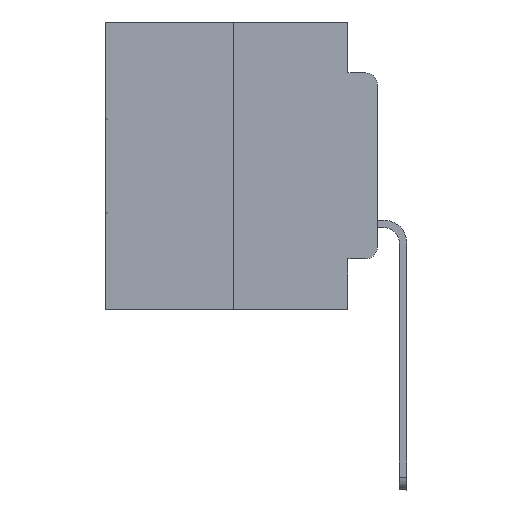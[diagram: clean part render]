
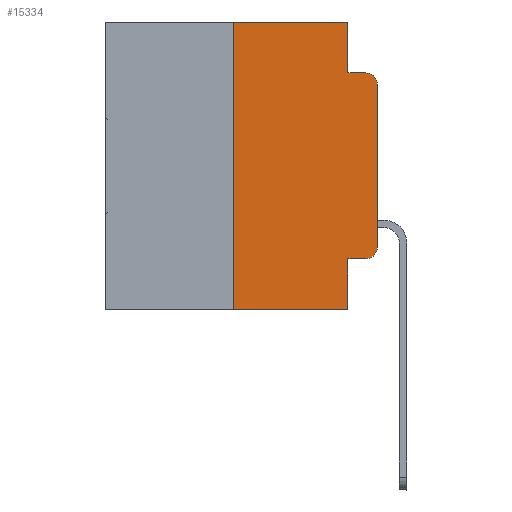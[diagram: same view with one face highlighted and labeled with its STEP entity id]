
A CAD part, left-side view. The second image highlights one B-rep face of the part: STEP entity #15334.
In plain terms, the highlighted planar face has unit normal (-1, 0, 0).
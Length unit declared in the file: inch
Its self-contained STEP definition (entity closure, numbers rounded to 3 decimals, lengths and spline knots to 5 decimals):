
#325 = AXIS2_PLACEMENT_3D ( 'NONE', #27544, #16345, #9337 ) ;
#445 = DIRECTION ( 'NONE',  ( 0., 0., -1. ) ) ;
#854 = CARTESIAN_POINT ( 'NONE',  ( 0., 0.051, -0.0885 ) ) ;
#1113 = DIRECTION ( 'NONE',  ( 1., 0., 0. ) ) ;
#1125 = VECTOR ( 'NONE', #6802, 39.37008 ) ;
#1430 = DIRECTION ( 'NONE',  ( 0., 0., -1. ) ) ;
#1581 = LINE ( 'NONE', #15450, #1125 ) ;
#1852 = VECTOR ( 'NONE', #19676, 39.37008 ) ;
#1858 = VECTOR ( 'NONE', #2871, 39.37008 ) ;
#1973 = CARTESIAN_POINT ( 'NONE',  ( 0., 0.051, -0.4115 ) ) ;
#2155 = EDGE_CURVE ( 'NONE', #29068, #17212, #22130, .T. ) ;
#2298 = EDGE_CURVE ( 'NONE', #24564, #20681, #26079, .T. ) ;
#2871 = DIRECTION ( 'NONE',  ( 0., -1., 0. ) ) ;
#3515 = PLANE ( 'NONE',  #11092 ) ;
#4290 = LINE ( 'NONE', #15476, #1852 ) ;
#4856 = DIRECTION ( 'NONE',  ( 0., -1., 0. ) ) ;
#5271 = CARTESIAN_POINT ( 'NONE',  ( 0., 0.02, -0.0885 ) ) ;
#5399 = CARTESIAN_POINT ( 'NONE',  ( 0., 0.051, -0.4115 ) ) ;
#5441 = CARTESIAN_POINT ( 'NONE',  ( 0., 0.25, -0.5 ) ) ;
#5605 = VECTOR ( 'NONE', #4856, 39.37008 ) ;
#6640 = EDGE_CURVE ( 'NONE', #12222, #18406, #27238, .T. ) ;
#6689 = EDGE_CURVE ( 'NONE', #25036, #13129, #12279, .T. ) ;
#6758 = VERTEX_POINT ( 'NONE', #5441 ) ;
#6802 = DIRECTION ( 'NONE',  ( 0., 0., -1. ) ) ;
#7118 = ORIENTED_EDGE ( 'NONE', *, *, #20360, .T. ) ;
#7338 = LINE ( 'NONE', #5399, #1858 ) ;
#7473 = ORIENTED_EDGE ( 'NONE', *, *, #18368, .F. ) ;
#7517 = CARTESIAN_POINT ( 'NONE',  ( 0., 0.473, -0.5 ) ) ;
#7795 = LINE ( 'NONE', #7517, #13905 ) ;
#8015 = CARTESIAN_POINT ( 'NONE',  ( 0., 0.051, 0. ) ) ;
#8665 = DIRECTION ( 'NONE',  ( 0., 0., -1. ) ) ;
#8822 = ORIENTED_EDGE ( 'NONE', *, *, #6640, .F. ) ;
#9126 = DIRECTION ( 'NONE',  ( 0., -1., 0. ) ) ;
#9337 = DIRECTION ( 'NONE',  ( 0., 0., -1. ) ) ;
#9690 = EDGE_CURVE ( 'NONE', #6758, #12222, #4290, .T. ) ;
#9694 = CARTESIAN_POINT ( 'NONE',  ( 0., 0.25, 0. ) ) ;
#9730 = CARTESIAN_POINT ( 'NONE',  ( 0., 0., -0.3915 ) ) ;
#11092 = AXIS2_PLACEMENT_3D ( 'NONE', #22046, #1113, #1430 ) ;
#11258 = AXIS2_PLACEMENT_3D ( 'NONE', #22275, #29105, #8665 ) ;
#11590 = CARTESIAN_POINT ( 'NONE',  ( 0., 0., -0.1085 ) ) ;
#11609 = VECTOR ( 'NONE', #9126, 39.37008 ) ;
#12222 = VERTEX_POINT ( 'NONE', #9694 ) ;
#12279 = CIRCLE ( 'NONE', #325, 0.02 ) ;
#12845 = ORIENTED_EDGE ( 'NONE', *, *, #20061, .T. ) ;
#13129 = VERTEX_POINT ( 'NONE', #9730 ) ;
#13905 = VECTOR ( 'NONE', #14505, 39.37008 ) ;
#13957 = CARTESIAN_POINT ( 'NONE',  ( 0., 0.051, -0.5 ) ) ;
#14182 = CARTESIAN_POINT ( 'NONE',  ( 0., 0., 0. ) ) ;
#14505 = DIRECTION ( 'NONE',  ( 0., -1., 0. ) ) ;
#14585 = VECTOR ( 'NONE', #28053, 39.37008 ) ;
#15334 = ADVANCED_FACE ( 'NONE', ( #19793 ), #3515, .F. ) ;
#15450 = CARTESIAN_POINT ( 'NONE',  ( 0., 0.051, 0. ) ) ;
#15452 = EDGE_CURVE ( 'NONE', #6758, #20681, #7795, .T. ) ;
#15476 = CARTESIAN_POINT ( 'NONE',  ( 0., 0.25, 0. ) ) ;
#15900 = CARTESIAN_POINT ( 'NONE',  ( 0., 0.473, 0. ) ) ;
#16345 = DIRECTION ( 'NONE',  ( -1., 0., 0. ) ) ;
#16535 = ORIENTED_EDGE ( 'NONE', *, *, #6689, .T. ) ;
#16761 = ORIENTED_EDGE ( 'NONE', *, *, #2298, .F. ) ;
#17212 = VERTEX_POINT ( 'NONE', #5271 ) ;
#18340 = VECTOR ( 'NONE', #445, 39.37008 ) ;
#18368 = EDGE_CURVE ( 'NONE', #18406, #29068, #1581, .T. ) ;
#18406 = VERTEX_POINT ( 'NONE', #29183 ) ;
#18711 = ORIENTED_EDGE ( 'NONE', *, *, #24608, .T. ) ;
#19676 = DIRECTION ( 'NONE',  ( 0., 0., 1. ) ) ;
#19793 = FACE_OUTER_BOUND ( 'NONE', #28825, .T. ) ;
#20061 = EDGE_CURVE ( 'NONE', #29197, #17212, #24132, .T. ) ;
#20360 = EDGE_CURVE ( 'NONE', #13129, #29197, #25678, .T. ) ;
#20681 = VERTEX_POINT ( 'NONE', #13957 ) ;
#22046 = CARTESIAN_POINT ( 'NONE',  ( 0., 0.473, 0. ) ) ;
#22130 = LINE ( 'NONE', #854, #11609 ) ;
#22275 = CARTESIAN_POINT ( 'NONE',  ( 0., 0.02, -0.1085 ) ) ;
#22353 = CARTESIAN_POINT ( 'NONE',  ( 0., 0.051, -0.0885 ) ) ;
#23962 = ORIENTED_EDGE ( 'NONE', *, *, #15452, .T. ) ;
#24132 = CIRCLE ( 'NONE', #11258, 0.02 ) ;
#24564 = VERTEX_POINT ( 'NONE', #1973 ) ;
#24608 = EDGE_CURVE ( 'NONE', #24564, #25036, #7338, .T. ) ;
#25036 = VERTEX_POINT ( 'NONE', #25802 ) ;
#25220 = ORIENTED_EDGE ( 'NONE', *, *, #2155, .F. ) ;
#25678 = LINE ( 'NONE', #14182, #14585 ) ;
#25802 = CARTESIAN_POINT ( 'NONE',  ( 0., 0.02, -0.4115 ) ) ;
#26079 = LINE ( 'NONE', #8015, #18340 ) ;
#27238 = LINE ( 'NONE', #15900, #5605 ) ;
#27544 = CARTESIAN_POINT ( 'NONE',  ( 0., 0.02, -0.3915 ) ) ;
#28036 = ORIENTED_EDGE ( 'NONE', *, *, #9690, .F. ) ;
#28053 = DIRECTION ( 'NONE',  ( 0., 0., 1. ) ) ;
#28825 = EDGE_LOOP ( 'NONE', ( #7118, #12845, #25220, #7473, #8822, #28036, #23962, #16761, #18711, #16535 ) ) ;
#29068 = VERTEX_POINT ( 'NONE', #22353 ) ;
#29105 = DIRECTION ( 'NONE',  ( -1., 0., 0. ) ) ;
#29183 = CARTESIAN_POINT ( 'NONE',  ( 0., 0.051, 0. ) ) ;
#29197 = VERTEX_POINT ( 'NONE', #11590 ) ;
